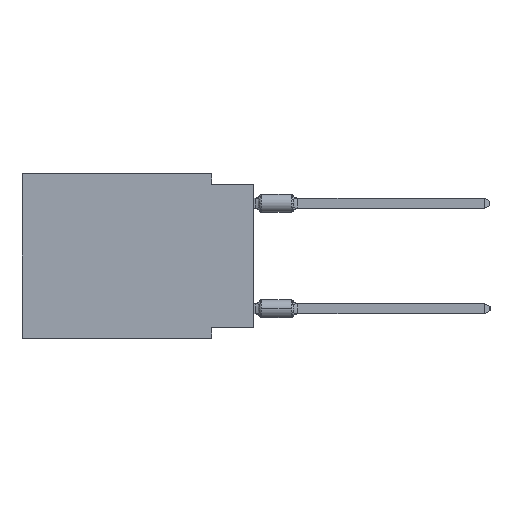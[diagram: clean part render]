
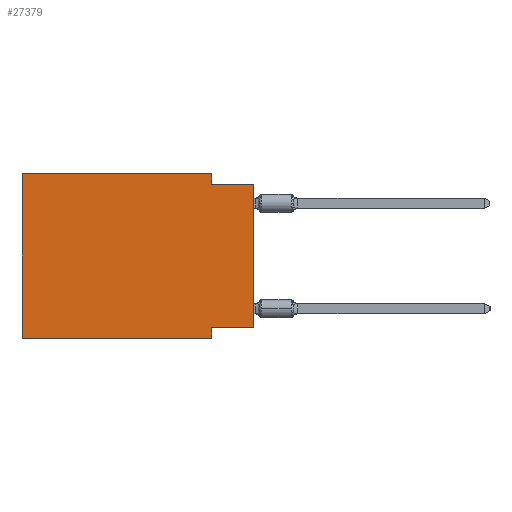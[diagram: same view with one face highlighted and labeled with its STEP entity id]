
A CAD part, left-side view. The second image highlights one B-rep face of the part: STEP entity #27379.
In plain terms, the highlighted planar face has unit normal (-1, 0, 0).
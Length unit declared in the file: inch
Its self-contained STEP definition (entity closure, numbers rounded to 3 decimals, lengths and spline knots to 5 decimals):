
#550 = VECTOR ( 'NONE', #32997, 39.37008 ) ;
#1800 = CARTESIAN_POINT ( 'NONE',  ( 0., 0., -0.365 ) ) ;
#3486 = EDGE_CURVE ( 'NONE', #38745, #34002, #30203, .T. ) ;
#3697 = EDGE_CURVE ( 'NONE', #51042, #48102, #6471, .T. ) ;
#3970 = CARTESIAN_POINT ( 'NONE',  ( 0., 0.55, 0. ) ) ;
#4938 = CARTESIAN_POINT ( 'NONE',  ( 0., 0.1, -0.39 ) ) ;
#5458 = ORIENTED_EDGE ( 'NONE', *, *, #22638, .F. ) ;
#5994 = EDGE_CURVE ( 'NONE', #45131, #38745, #18235, .T. ) ;
#6471 = LINE ( 'NONE', #45571, #550 ) ;
#7412 = EDGE_CURVE ( 'NONE', #54921, #41602, #28473, .T. ) ;
#9713 = VECTOR ( 'NONE', #35305, 39.37008 ) ;
#11250 = CARTESIAN_POINT ( 'NONE',  ( 0., 0.55, 0. ) ) ;
#12627 = DIRECTION ( 'NONE',  ( 0., -1., 0. ) ) ;
#13309 = VECTOR ( 'NONE', #12627, 39.37008 ) ;
#13742 = VECTOR ( 'NONE', #49174, 39.37008 ) ;
#14501 = LINE ( 'NONE', #32468, #41699 ) ;
#15171 = EDGE_CURVE ( 'NONE', #45131, #41602, #56333, .T. ) ;
#17826 = VECTOR ( 'NONE', #34507, 39.37008 ) ;
#17958 = CARTESIAN_POINT ( 'NONE',  ( 0., 0.55, 0. ) ) ;
#18192 = CARTESIAN_POINT ( 'NONE',  ( 0., 0.55, 0. ) ) ;
#18235 = LINE ( 'NONE', #17958, #44991 ) ;
#19904 = CARTESIAN_POINT ( 'NONE',  ( 0., 0.1, -0.025 ) ) ;
#22147 = LINE ( 'NONE', #53556, #9713 ) ;
#22638 = EDGE_CURVE ( 'NONE', #51042, #54921, #49445, .T. ) ;
#23281 = EDGE_CURVE ( 'NONE', #45917, #48102, #22147, .T. ) ;
#23659 = ORIENTED_EDGE ( 'NONE', *, *, #23281, .F. ) ;
#24452 = DIRECTION ( 'NONE',  ( 0., 0., -1. ) ) ;
#27379 = ADVANCED_FACE ( 'NONE', ( #37237 ), #32943, .F. ) ;
#28473 = LINE ( 'NONE', #4938, #53347 ) ;
#28645 = DIRECTION ( 'NONE',  ( 1., 0., 0. ) ) ;
#30203 = LINE ( 'NONE', #3970, #17826 ) ;
#30326 = CARTESIAN_POINT ( 'NONE',  ( 0., 0.55, -0.39 ) ) ;
#32468 = CARTESIAN_POINT ( 'NONE',  ( 0., 0.1, 0. ) ) ;
#32943 = PLANE ( 'NONE',  #39961 ) ;
#32997 = DIRECTION ( 'NONE',  ( 0., 0., 1. ) ) ;
#33472 = ORIENTED_EDGE ( 'NONE', *, *, #55457, .F. ) ;
#34002 = VERTEX_POINT ( 'NONE', #55429 ) ;
#34507 = DIRECTION ( 'NONE',  ( 0., -1., 0. ) ) ;
#35114 = EDGE_LOOP ( 'NONE', ( #54029, #23659, #33472, #47799, #45087, #44963, #53976, #5458 ) ) ;
#35305 = DIRECTION ( 'NONE',  ( 0., -1., 0. ) ) ;
#35671 = DIRECTION ( 'NONE',  ( 0., 0., 1. ) ) ;
#37237 = FACE_OUTER_BOUND ( 'NONE', #35114, .T. ) ;
#38745 = VERTEX_POINT ( 'NONE', #18192 ) ;
#39961 = AXIS2_PLACEMENT_3D ( 'NONE', #11250, #28645, #50647 ) ;
#40002 = DIRECTION ( 'NONE',  ( 0., 0., -1. ) ) ;
#41602 = VERTEX_POINT ( 'NONE', #45540 ) ;
#41699 = VECTOR ( 'NONE', #24452, 39.37008 ) ;
#42064 = CARTESIAN_POINT ( 'NONE',  ( 0., 0., -0.365 ) ) ;
#44963 = ORIENTED_EDGE ( 'NONE', *, *, #15171, .T. ) ;
#44991 = VECTOR ( 'NONE', #35671, 39.37008 ) ;
#45087 = ORIENTED_EDGE ( 'NONE', *, *, #5994, .F. ) ;
#45131 = VERTEX_POINT ( 'NONE', #54689 ) ;
#45540 = CARTESIAN_POINT ( 'NONE',  ( 0., 0.1, -0.39 ) ) ;
#45571 = CARTESIAN_POINT ( 'NONE',  ( 0., 0., 0. ) ) ;
#45917 = VERTEX_POINT ( 'NONE', #19904 ) ;
#47799 = ORIENTED_EDGE ( 'NONE', *, *, #3486, .F. ) ;
#48102 = VERTEX_POINT ( 'NONE', #56349 ) ;
#49174 = DIRECTION ( 'NONE',  ( 0., 1., 0. ) ) ;
#49445 = LINE ( 'NONE', #1800, #13742 ) ;
#50647 = DIRECTION ( 'NONE',  ( 0., 0., -1. ) ) ;
#51042 = VERTEX_POINT ( 'NONE', #42064 ) ;
#53347 = VECTOR ( 'NONE', #40002, 39.37008 ) ;
#53556 = CARTESIAN_POINT ( 'NONE',  ( 0., 0., -0.025 ) ) ;
#53976 = ORIENTED_EDGE ( 'NONE', *, *, #7412, .F. ) ;
#54029 = ORIENTED_EDGE ( 'NONE', *, *, #3697, .T. ) ;
#54689 = CARTESIAN_POINT ( 'NONE',  ( 0., 0.55, -0.39 ) ) ;
#54921 = VERTEX_POINT ( 'NONE', #56383 ) ;
#55429 = CARTESIAN_POINT ( 'NONE',  ( 0., 0.1, 0. ) ) ;
#55457 = EDGE_CURVE ( 'NONE', #34002, #45917, #14501, .T. ) ;
#56333 = LINE ( 'NONE', #30326, #13309 ) ;
#56349 = CARTESIAN_POINT ( 'NONE',  ( 0., 0., -0.025 ) ) ;
#56383 = CARTESIAN_POINT ( 'NONE',  ( 0., 0.1, -0.365 ) ) ;
